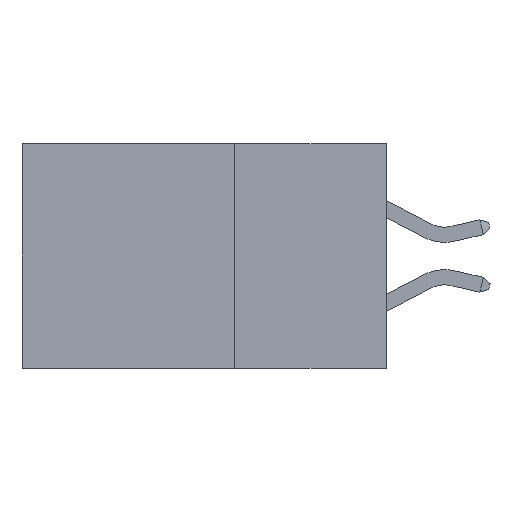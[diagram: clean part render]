
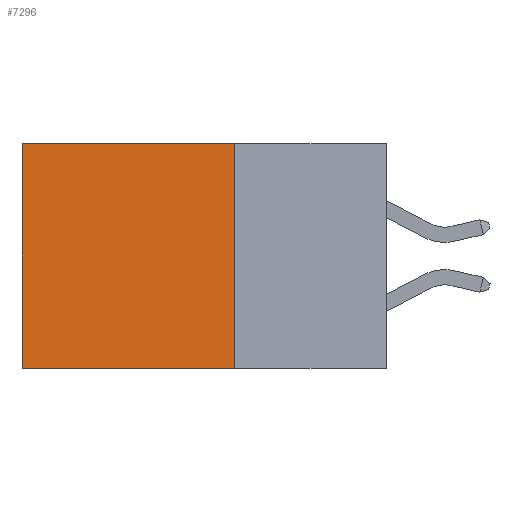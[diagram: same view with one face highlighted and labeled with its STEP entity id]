
A CAD part, left-side view. The second image highlights one B-rep face of the part: STEP entity #7296.
In plain terms, the highlighted planar face has unit normal (-1, 0, 0).
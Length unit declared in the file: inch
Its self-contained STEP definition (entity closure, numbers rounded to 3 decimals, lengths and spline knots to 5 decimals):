
#193 = EDGE_CURVE ( 'NONE', #5759, #1024, #18130, .T. ) ;
#947 = VECTOR ( 'NONE', #2874, 39.37008 ) ;
#1024 = VERTEX_POINT ( 'NONE', #16837 ) ;
#1213 = CARTESIAN_POINT ( 'NONE',  ( 0.298, 0.6, -0.37 ) ) ;
#1243 = LINE ( 'NONE', #14720, #16095 ) ;
#1447 = LINE ( 'NONE', #4263, #947 ) ;
#2132 = EDGE_CURVE ( 'NONE', #5759, #19045, #1447, .T. ) ;
#2874 = DIRECTION ( 'NONE',  ( 0., 1., 0. ) ) ;
#3466 = CARTESIAN_POINT ( 'NONE',  ( 0.298, 0.6, 0. ) ) ;
#4263 = CARTESIAN_POINT ( 'NONE',  ( 0.298, 0.25, 0. ) ) ;
#5223 = DIRECTION ( 'NONE',  ( 0., 0., -1. ) ) ;
#5298 = ORIENTED_EDGE ( 'NONE', *, *, #7100, .T. ) ;
#5759 = VERTEX_POINT ( 'NONE', #14228 ) ;
#5886 = EDGE_LOOP ( 'NONE', ( #5298, #11649, #12944, #15568 ) ) ;
#6930 = CARTESIAN_POINT ( 'NONE',  ( 0.298, 0.25, -0.37 ) ) ;
#7100 = EDGE_CURVE ( 'NONE', #19045, #11207, #1243, .T. ) ;
#7296 = ADVANCED_FACE ( 'NONE', ( #10634 ), #13068, .F. ) ;
#8544 = CARTESIAN_POINT ( 'NONE',  ( 0.298, 0.25, 0. ) ) ;
#8786 = CARTESIAN_POINT ( 'NONE',  ( 0.298, 0.25, 0. ) ) ;
#9969 = AXIS2_PLACEMENT_3D ( 'NONE', #8544, #19474, #16205 ) ;
#10634 = FACE_OUTER_BOUND ( 'NONE', #5886, .T. ) ;
#11207 = VERTEX_POINT ( 'NONE', #1213 ) ;
#11649 = ORIENTED_EDGE ( 'NONE', *, *, #12585, .F. ) ;
#12585 = EDGE_CURVE ( 'NONE', #1024, #11207, #13089, .T. ) ;
#12944 = ORIENTED_EDGE ( 'NONE', *, *, #193, .F. ) ;
#13068 = PLANE ( 'NONE',  #9969 ) ;
#13089 = LINE ( 'NONE', #6930, #16829 ) ;
#14228 = CARTESIAN_POINT ( 'NONE',  ( 0.298, 0.25, 0. ) ) ;
#14720 = CARTESIAN_POINT ( 'NONE',  ( 0.298, 0.6, 0. ) ) ;
#15568 = ORIENTED_EDGE ( 'NONE', *, *, #2132, .T. ) ;
#16095 = VECTOR ( 'NONE', #5223, 39.37008 ) ;
#16205 = DIRECTION ( 'NONE',  ( 0., 0., -1. ) ) ;
#16630 = VECTOR ( 'NONE', #18063, 39.37008 ) ;
#16829 = VECTOR ( 'NONE', #18214, 39.37008 ) ;
#16837 = CARTESIAN_POINT ( 'NONE',  ( 0.298, 0.25, -0.37 ) ) ;
#18063 = DIRECTION ( 'NONE',  ( 0., 0., -1. ) ) ;
#18130 = LINE ( 'NONE', #8786, #16630 ) ;
#18214 = DIRECTION ( 'NONE',  ( 0., 1., 0. ) ) ;
#19045 = VERTEX_POINT ( 'NONE', #3466 ) ;
#19474 = DIRECTION ( 'NONE',  ( 1., 0., 0. ) ) ;
